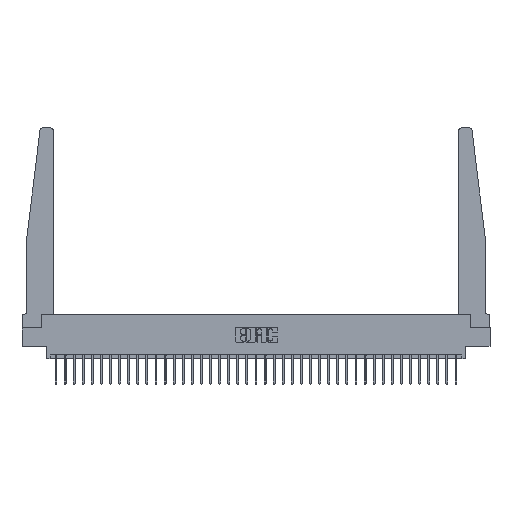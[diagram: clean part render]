
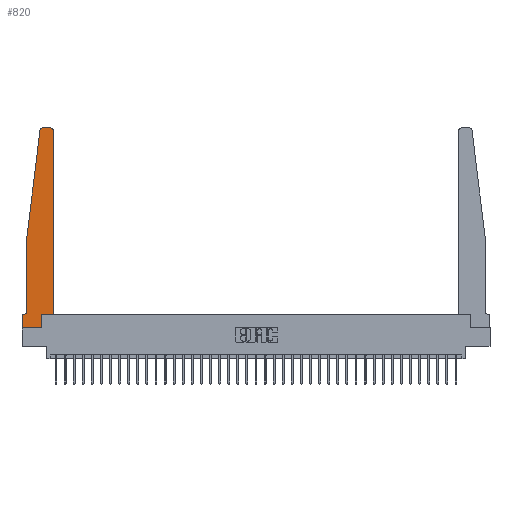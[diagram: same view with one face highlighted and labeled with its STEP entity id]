
A CAD part, top view. The second image highlights one B-rep face of the part: STEP entity #820.
In plain terms, the highlighted planar face has unit normal (0, 0, 1).
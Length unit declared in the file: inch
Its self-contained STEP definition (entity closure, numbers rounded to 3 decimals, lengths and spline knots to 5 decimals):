
#715 = LINE ( 'NONE', #11344, #11010 ) ;
#795 = LINE ( 'NONE', #27898, #8103 ) ;
#820 = ADVANCED_FACE ( 'NONE', ( #26327 ), #5494, .T. ) ;
#2087 = DIRECTION ( 'NONE',  ( 0., -1., 0. ) ) ;
#2336 = EDGE_CURVE ( 'NONE', #9358, #17822, #15674, .T. ) ;
#2495 = CIRCLE ( 'NONE', #19715, 0.05 ) ;
#2548 = VECTOR ( 'NONE', #12403, 39.37008 ) ;
#2747 = EDGE_CURVE ( 'NONE', #30690, #27464, #2495, .T. ) ;
#2837 = ORIENTED_EDGE ( 'NONE', *, *, #17303, .T. ) ;
#2952 = EDGE_CURVE ( 'NONE', #11793, #30690, #12572, .T. ) ;
#3120 = ORIENTED_EDGE ( 'NONE', *, *, #3706, .T. ) ;
#3706 = EDGE_CURVE ( 'NONE', #29215, #11793, #795, .T. ) ;
#4224 = CARTESIAN_POINT ( 'NONE',  ( 0., 0.1875, 0.37 ) ) ;
#4369 = CARTESIAN_POINT ( 'NONE',  ( 0.27653, 2.75, 0.37 ) ) ;
#4623 = EDGE_CURVE ( 'NONE', #27464, #25701, #715, .T. ) ;
#4739 = VECTOR ( 'NONE', #10342, 39.37008 ) ;
#4755 = CARTESIAN_POINT ( 'NONE',  ( 0.065, 1.25, 0.37 ) ) ;
#5455 = LINE ( 'NONE', #31867, #4739 ) ;
#5494 = PLANE ( 'NONE',  #12246 ) ;
#6380 = LINE ( 'NONE', #9164, #33582 ) ;
#6639 = DIRECTION ( 'NONE',  ( 0., 1., 0. ) ) ;
#7089 = CARTESIAN_POINT ( 'NONE',  ( 0.2605, 0.18, 0.37 ) ) ;
#7415 = ORIENTED_EDGE ( 'NONE', *, *, #23365, .T. ) ;
#7571 = ORIENTED_EDGE ( 'NONE', *, *, #2336, .T. ) ;
#7776 = EDGE_CURVE ( 'NONE', #25701, #14238, #7985, .T. ) ;
#7985 = LINE ( 'NONE', #26564, #21823 ) ;
#8048 = CARTESIAN_POINT ( 'NONE',  ( 0.015, 0.1875, 0.37 ) ) ;
#8103 = VECTOR ( 'NONE', #22339, 39.37008 ) ;
#8940 = CARTESIAN_POINT ( 'NONE',  ( 0.015, 0.2375, 0.37 ) ) ;
#9164 = CARTESIAN_POINT ( 'NONE',  ( 0.425, 0.18, 0.37 ) ) ;
#9324 = ORIENTED_EDGE ( 'NONE', *, *, #14222, .T. ) ;
#9358 = VERTEX_POINT ( 'NONE', #16475 ) ;
#10185 = AXIS2_PLACEMENT_3D ( 'NONE', #30191, #30014, #16773 ) ;
#10279 = VERTEX_POINT ( 'NONE', #4369 ) ;
#10342 = DIRECTION ( 'NONE',  ( 0., 1., 0. ) ) ;
#10376 = DIRECTION ( 'NONE',  ( 0., 0., 1. ) ) ;
#10792 = EDGE_LOOP ( 'NONE', ( #2837, #7415, #3120, #25495, #16614, #33045, #21818, #22779, #9324, #13315, #19836, #7571 ) ) ;
#10892 = DIRECTION ( 'NONE',  ( 1., 0., 0. ) ) ;
#11010 = VECTOR ( 'NONE', #21744, 39.37008 ) ;
#11344 = CARTESIAN_POINT ( 'NONE',  ( 0.065, 0.1875, 0.37 ) ) ;
#11610 = VECTOR ( 'NONE', #25874, 39.37008 ) ;
#11793 = VERTEX_POINT ( 'NONE', #4755 ) ;
#11860 = LINE ( 'NONE', #14955, #12284 ) ;
#11879 = DIRECTION ( 'NONE',  ( 0., 0., 1. ) ) ;
#12207 = EDGE_CURVE ( 'NONE', #16539, #9358, #11860, .T. ) ;
#12246 = AXIS2_PLACEMENT_3D ( 'NONE', #34152, #10376, #10892 ) ;
#12284 = VECTOR ( 'NONE', #6639, 39.37008 ) ;
#12403 = DIRECTION ( 'NONE',  ( 0., -1., 0. ) ) ;
#12572 = LINE ( 'NONE', #20365, #2548 ) ;
#12806 = CARTESIAN_POINT ( 'NONE',  ( 0.065, 0.2375, 0.37 ) ) ;
#13153 = LINE ( 'NONE', #13326, #14688 ) ;
#13315 = ORIENTED_EDGE ( 'NONE', *, *, #17522, .T. ) ;
#13326 = CARTESIAN_POINT ( 'NONE',  ( 0.25, 2.75, 0.37 ) ) ;
#14222 = EDGE_CURVE ( 'NONE', #24644, #27976, #5455, .T. ) ;
#14238 = VERTEX_POINT ( 'NONE', #33073 ) ;
#14688 = VECTOR ( 'NONE', #26697, 39.37008 ) ;
#14955 = CARTESIAN_POINT ( 'NONE',  ( 0.425, 0.18, 0.37 ) ) ;
#15674 = CIRCLE ( 'NONE', #10185, 0.03 ) ;
#16475 = CARTESIAN_POINT ( 'NONE',  ( 0.425, 2.72, 0.37 ) ) ;
#16539 = VERTEX_POINT ( 'NONE', #18870 ) ;
#16614 = ORIENTED_EDGE ( 'NONE', *, *, #2747, .T. ) ;
#16773 = DIRECTION ( 'NONE',  ( 1., 0., 0. ) ) ;
#17303 = EDGE_CURVE ( 'NONE', #17822, #10279, #13153, .T. ) ;
#17522 = EDGE_CURVE ( 'NONE', #27976, #16539, #6380, .T. ) ;
#17822 = VERTEX_POINT ( 'NONE', #33043 ) ;
#18870 = CARTESIAN_POINT ( 'NONE',  ( 0.425, 0.18, 0.37 ) ) ;
#19715 = AXIS2_PLACEMENT_3D ( 'NONE', #8940, #22297, #32392 ) ;
#19738 = DIRECTION ( 'NONE',  ( 1., 0., 0. ) ) ;
#19836 = ORIENTED_EDGE ( 'NONE', *, *, #12207, .T. ) ;
#20365 = CARTESIAN_POINT ( 'NONE',  ( 0.065, 1.25, 0.37 ) ) ;
#20977 = LINE ( 'NONE', #31126, #11610 ) ;
#21744 = DIRECTION ( 'NONE',  ( -1., 0., 0. ) ) ;
#21818 = ORIENTED_EDGE ( 'NONE', *, *, #7776, .T. ) ;
#21823 = VECTOR ( 'NONE', #2087, 39.37008 ) ;
#22297 = DIRECTION ( 'NONE',  ( 0., 0., -1. ) ) ;
#22339 = DIRECTION ( 'NONE',  ( -0.122, -0.992, 0. ) ) ;
#22779 = ORIENTED_EDGE ( 'NONE', *, *, #24027, .T. ) ;
#23365 = EDGE_CURVE ( 'NONE', #10279, #29215, #33772, .T. ) ;
#24027 = EDGE_CURVE ( 'NONE', #14238, #24644, #20977, .T. ) ;
#24644 = VERTEX_POINT ( 'NONE', #27897 ) ;
#25495 = ORIENTED_EDGE ( 'NONE', *, *, #2952, .T. ) ;
#25701 = VERTEX_POINT ( 'NONE', #4224 ) ;
#25874 = DIRECTION ( 'NONE',  ( 1., 0., 0. ) ) ;
#26327 = FACE_OUTER_BOUND ( 'NONE', #10792, .T. ) ;
#26564 = CARTESIAN_POINT ( 'NONE',  ( 0., 0., 0.37 ) ) ;
#26697 = DIRECTION ( 'NONE',  ( -1., 0., 0. ) ) ;
#27464 = VERTEX_POINT ( 'NONE', #8048 ) ;
#27658 = AXIS2_PLACEMENT_3D ( 'NONE', #27851, #11879, #30312 ) ;
#27851 = CARTESIAN_POINT ( 'NONE',  ( 0.27653, 2.72, 0.37 ) ) ;
#27897 = CARTESIAN_POINT ( 'NONE',  ( 0.2605, 0., 0.37 ) ) ;
#27898 = CARTESIAN_POINT ( 'NONE',  ( 0.065, 1.25, 0.37 ) ) ;
#27976 = VERTEX_POINT ( 'NONE', #7089 ) ;
#29215 = VERTEX_POINT ( 'NONE', #29754 ) ;
#29754 = CARTESIAN_POINT ( 'NONE',  ( 0.24675, 2.72367, 0.37 ) ) ;
#30014 = DIRECTION ( 'NONE',  ( 0., 0., 1. ) ) ;
#30191 = CARTESIAN_POINT ( 'NONE',  ( 0.395, 2.72, 0.37 ) ) ;
#30312 = DIRECTION ( 'NONE',  ( 1., 0., 0. ) ) ;
#30690 = VERTEX_POINT ( 'NONE', #12806 ) ;
#31126 = CARTESIAN_POINT ( 'NONE',  ( 0., 0., 0.37 ) ) ;
#31867 = CARTESIAN_POINT ( 'NONE',  ( 0.2605, 0.18, 0.37 ) ) ;
#32392 = DIRECTION ( 'NONE',  ( -1., 0., 0. ) ) ;
#33043 = CARTESIAN_POINT ( 'NONE',  ( 0.395, 2.75, 0.37 ) ) ;
#33045 = ORIENTED_EDGE ( 'NONE', *, *, #4623, .T. ) ;
#33073 = CARTESIAN_POINT ( 'NONE',  ( 0., 0., 0.37 ) ) ;
#33582 = VECTOR ( 'NONE', #19738, 39.37008 ) ;
#33772 = CIRCLE ( 'NONE', #27658, 0.03 ) ;
#34152 = CARTESIAN_POINT ( 'NONE',  ( 0., 0.1875, 0.37 ) ) ;
